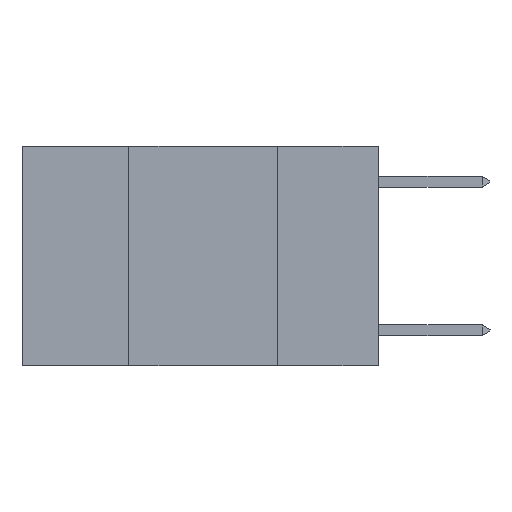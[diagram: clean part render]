
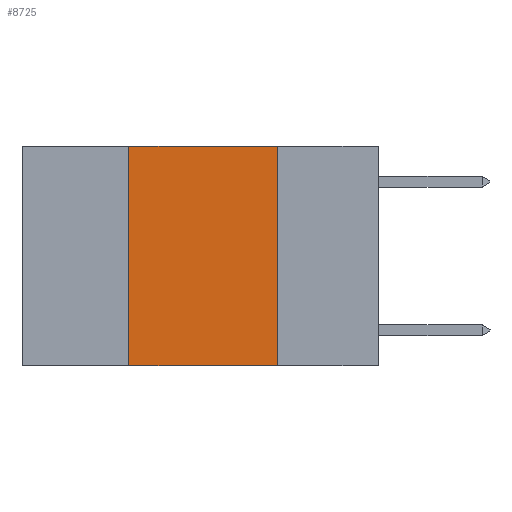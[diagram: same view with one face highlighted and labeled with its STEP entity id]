
A CAD part, left-side view. The second image highlights one B-rep face of the part: STEP entity #8725.
In plain terms, the highlighted planar face has unit normal (-1, 0, 0).
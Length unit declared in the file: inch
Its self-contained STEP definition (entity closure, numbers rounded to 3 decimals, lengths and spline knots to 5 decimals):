
#242 = DIRECTION ( 'NONE',  ( 0., 0., 1. ) ) ;
#291 = CARTESIAN_POINT ( 'NONE',  ( 0., 0.42, 0. ) ) ;
#1390 = CARTESIAN_POINT ( 'NONE',  ( 0., 0.17, 0. ) ) ;
#4387 = EDGE_CURVE ( 'NONE', #8240, #13936, #20658, .T. ) ;
#5419 = DIRECTION ( 'NONE',  ( 0., 0., -1. ) ) ;
#5454 = DIRECTION ( 'NONE',  ( 1., 0., 0. ) ) ;
#5503 = PLANE ( 'NONE',  #16818 ) ;
#5647 = FACE_OUTER_BOUND ( 'NONE', #18064, .T. ) ;
#5806 = CARTESIAN_POINT ( 'NONE',  ( 0., 0.6, 0. ) ) ;
#8042 = VERTEX_POINT ( 'NONE', #1390 ) ;
#8240 = VERTEX_POINT ( 'NONE', #10178 ) ;
#8725 = ADVANCED_FACE ( 'NONE', ( #5647 ), #5503, .F. ) ;
#9836 = VERTEX_POINT ( 'NONE', #10173 ) ;
#10173 = CARTESIAN_POINT ( 'NONE',  ( 0., 0.17, -0.37 ) ) ;
#10178 = CARTESIAN_POINT ( 'NONE',  ( 0., 0.42, -0.37 ) ) ;
#10441 = CARTESIAN_POINT ( 'NONE',  ( 0., 0.42, 0. ) ) ;
#10575 = CARTESIAN_POINT ( 'NONE',  ( 0., 0.6, -0.37 ) ) ;
#10746 = EDGE_CURVE ( 'NONE', #8240, #9836, #20690, .T. ) ;
#11183 = VECTOR ( 'NONE', #19968, 39.37008 ) ;
#11227 = EDGE_CURVE ( 'NONE', #13936, #8042, #17740, .T. ) ;
#11231 = LINE ( 'NONE', #18220, #11183 ) ;
#11560 = DIRECTION ( 'NONE',  ( 0., -1., 0. ) ) ;
#13936 = VERTEX_POINT ( 'NONE', #10441 ) ;
#16344 = EDGE_CURVE ( 'NONE', #8042, #9836, #11231, .T. ) ;
#16818 = AXIS2_PLACEMENT_3D ( 'NONE', #5806, #5454, #5419 ) ;
#17671 = VECTOR ( 'NONE', #21982, 39.37008 ) ;
#17740 = LINE ( 'NONE', #20127, #17671 ) ;
#18064 = EDGE_LOOP ( 'NONE', ( #18289, #20394, #20467, #20911 ) ) ;
#18220 = CARTESIAN_POINT ( 'NONE',  ( 0., 0.17, 0. ) ) ;
#18289 = ORIENTED_EDGE ( 'NONE', *, *, #16344, .F. ) ;
#19968 = DIRECTION ( 'NONE',  ( 0., 0., -1. ) ) ;
#20127 = CARTESIAN_POINT ( 'NONE',  ( 0., 0.6, 0. ) ) ;
#20394 = ORIENTED_EDGE ( 'NONE', *, *, #11227, .F. ) ;
#20467 = ORIENTED_EDGE ( 'NONE', *, *, #4387, .F. ) ;
#20658 = LINE ( 'NONE', #291, #21166 ) ;
#20690 = LINE ( 'NONE', #10575, #20730 ) ;
#20730 = VECTOR ( 'NONE', #11560, 39.37008 ) ;
#20911 = ORIENTED_EDGE ( 'NONE', *, *, #10746, .T. ) ;
#21166 = VECTOR ( 'NONE', #242, 39.37008 ) ;
#21982 = DIRECTION ( 'NONE',  ( 0., -1., 0. ) ) ;
